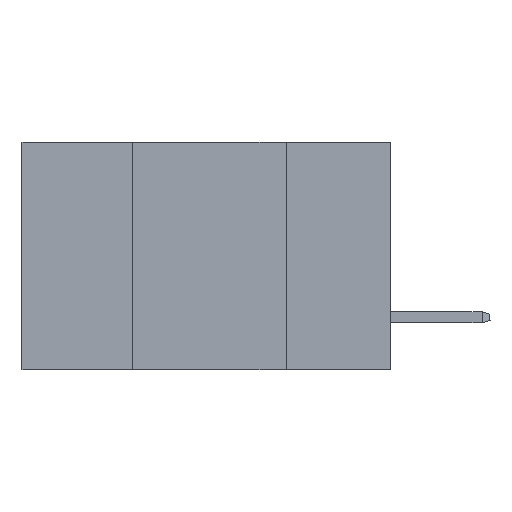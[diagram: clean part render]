
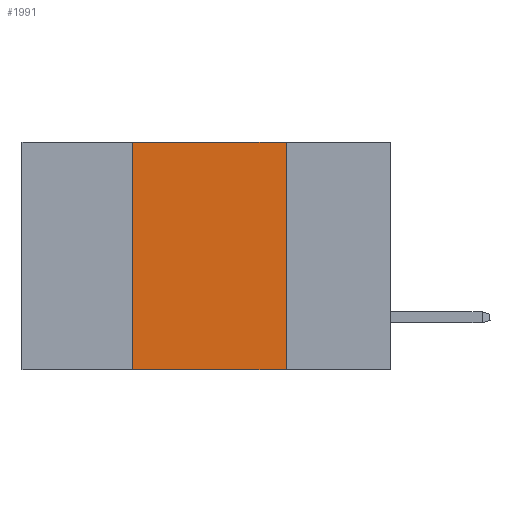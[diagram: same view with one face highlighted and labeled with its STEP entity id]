
A CAD part, left-side view. The second image highlights one B-rep face of the part: STEP entity #1991.
In plain terms, the highlighted planar face has unit normal (-1, 0, 0).
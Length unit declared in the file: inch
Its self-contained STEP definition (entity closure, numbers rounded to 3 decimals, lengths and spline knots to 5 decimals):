
#22 = CARTESIAN_POINT ( 'NONE',  ( 0., 0.17, 0. ) ) ;
#75 = LINE ( 'NONE', #3600, #10134 ) ;
#362 = DIRECTION ( 'NONE',  ( 1., 0., 0. ) ) ;
#703 = LINE ( 'NONE', #8156, #9108 ) ;
#1586 = EDGE_LOOP ( 'NONE', ( #10385, #1661, #10945, #7859 ) ) ;
#1661 = ORIENTED_EDGE ( 'NONE', *, *, #6463, .F. ) ;
#1833 = DIRECTION ( 'NONE',  ( 0., 0., -1. ) ) ;
#1991 = ADVANCED_FACE ( 'NONE', ( #5133 ), #4243, .F. ) ;
#3600 = CARTESIAN_POINT ( 'NONE',  ( 0., 0.42, 0. ) ) ;
#3689 = VERTEX_POINT ( 'NONE', #5139 ) ;
#4243 = PLANE ( 'NONE',  #8450 ) ;
#4249 = CARTESIAN_POINT ( 'NONE',  ( 0., 0.6, -0.37 ) ) ;
#4471 = EDGE_CURVE ( 'NONE', #10547, #7292, #11959, .T. ) ;
#4566 = DIRECTION ( 'NONE',  ( 0., 0., 1. ) ) ;
#4971 = CARTESIAN_POINT ( 'NONE',  ( 0., 0.42, -0.37 ) ) ;
#5133 = FACE_OUTER_BOUND ( 'NONE', #1586, .T. ) ;
#5139 = CARTESIAN_POINT ( 'NONE',  ( 0., 0.42, 0. ) ) ;
#6463 = EDGE_CURVE ( 'NONE', #3689, #12669, #703, .T. ) ;
#6768 = CARTESIAN_POINT ( 'NONE',  ( 0., 0.17, -0.37 ) ) ;
#7292 = VERTEX_POINT ( 'NONE', #6768 ) ;
#7339 = CARTESIAN_POINT ( 'NONE',  ( 0., 0.17, 0. ) ) ;
#7365 = VECTOR ( 'NONE', #9151, 39.37008 ) ;
#7859 = ORIENTED_EDGE ( 'NONE', *, *, #4471, .T. ) ;
#8018 = VECTOR ( 'NONE', #1833, 39.37008 ) ;
#8156 = CARTESIAN_POINT ( 'NONE',  ( 0., 0.6, 0. ) ) ;
#8325 = EDGE_CURVE ( 'NONE', #12669, #7292, #12638, .T. ) ;
#8448 = DIRECTION ( 'NONE',  ( 0., -1., 0. ) ) ;
#8450 = AXIS2_PLACEMENT_3D ( 'NONE', #8979, #362, #10950 ) ;
#8979 = CARTESIAN_POINT ( 'NONE',  ( 0., 0.6, 0. ) ) ;
#9075 = EDGE_CURVE ( 'NONE', #10547, #3689, #75, .T. ) ;
#9108 = VECTOR ( 'NONE', #8448, 39.37008 ) ;
#9151 = DIRECTION ( 'NONE',  ( 0., -1., 0. ) ) ;
#10134 = VECTOR ( 'NONE', #4566, 39.37008 ) ;
#10385 = ORIENTED_EDGE ( 'NONE', *, *, #8325, .F. ) ;
#10547 = VERTEX_POINT ( 'NONE', #4971 ) ;
#10945 = ORIENTED_EDGE ( 'NONE', *, *, #9075, .F. ) ;
#10950 = DIRECTION ( 'NONE',  ( 0., 0., -1. ) ) ;
#11959 = LINE ( 'NONE', #4249, #7365 ) ;
#12638 = LINE ( 'NONE', #22, #8018 ) ;
#12669 = VERTEX_POINT ( 'NONE', #7339 ) ;
